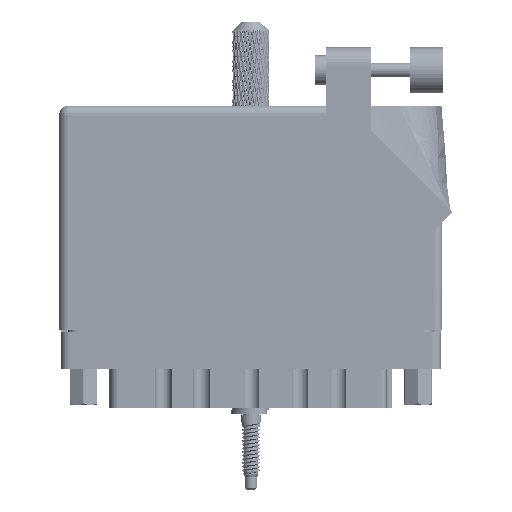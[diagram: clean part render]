
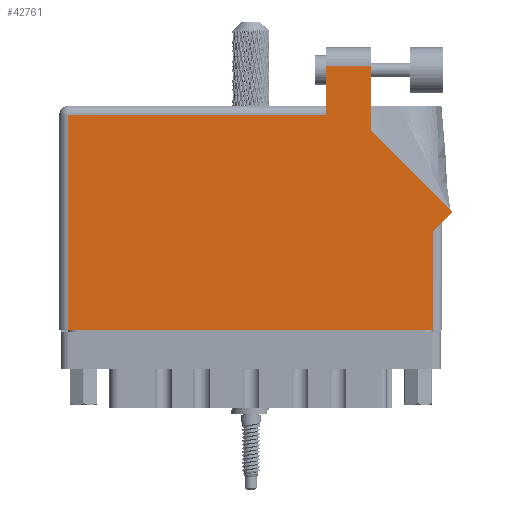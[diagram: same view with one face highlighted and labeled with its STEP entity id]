
A CAD part, front view. The second image highlights one B-rep face of the part: STEP entity #42761.
In plain terms, the highlighted face is planar.
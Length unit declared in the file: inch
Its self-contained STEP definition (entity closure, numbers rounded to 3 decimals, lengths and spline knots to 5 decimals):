
#889 = EDGE_CURVE ( 'NONE', #125285, #100103, #97054, .T. ) ;
#2261 = CARTESIAN_POINT ( 'NONE',  ( 0.062, 1.468, 0. ) ) ;
#2475 = DIRECTION ( 'NONE',  ( 0., -1., 0. ) ) ;
#2908 = CARTESIAN_POINT ( 'NONE',  ( 0.062, 0., 0. ) ) ;
#2923 = CARTESIAN_POINT ( 'NONE',  ( 2.55, 0.675, 0. ) ) ;
#3176 = CARTESIAN_POINT ( 'NONE',  ( 0., 1.53, 0. ) ) ;
#3602 = DIRECTION ( 'NONE',  ( -1., 0., 0. ) ) ;
#3746 = CARTESIAN_POINT ( 'NONE',  ( 1.819, 1.468, 0. ) ) ;
#4443 = CARTESIAN_POINT ( 'NONE',  ( 2.126, 1.36442, 0. ) ) ;
#5209 = DIRECTION ( 'NONE',  ( -0.707, 0.707, 0. ) ) ;
#12497 = LINE ( 'NONE', #119023, #41868 ) ;
#13631 = VECTOR ( 'NONE', #2475, 39.37008 ) ;
#15445 = LINE ( 'NONE', #98845, #117374 ) ;
#19598 = VECTOR ( 'NONE', #89529, 39.37008 ) ;
#20629 = DIRECTION ( 'NONE',  ( 0., 1., 0. ) ) ;
#27880 = LINE ( 'NONE', #84916, #81820 ) ;
#28435 = VERTEX_POINT ( 'NONE', #3746 ) ;
#29149 = EDGE_CURVE ( 'NONE', #54932, #73331, #53406, .T. ) ;
#33263 = VERTEX_POINT ( 'NONE', #53024 ) ;
#33855 = VERTEX_POINT ( 'NONE', #74916 ) ;
#35465 = CARTESIAN_POINT ( 'NONE',  ( 0., 1.468, 0. ) ) ;
#35721 = DIRECTION ( 'NONE',  ( 0.707, 0.707, 0. ) ) ;
#38159 = LINE ( 'NONE', #60083, #19598 ) ;
#38799 = ORIENTED_EDGE ( 'NONE', *, *, #50489, .T. ) ;
#39021 = LINE ( 'NONE', #52454, #88460 ) ;
#41401 = ORIENTED_EDGE ( 'NONE', *, *, #29149, .T. ) ;
#41868 = VECTOR ( 'NONE', #80626, 39.37008 ) ;
#42761 = ADVANCED_FACE ( 'NONE', ( #68547 ), #42949, .F. ) ;
#42949 = PLANE ( 'NONE',  #79005 ) ;
#49783 = VERTEX_POINT ( 'NONE', #2923 ) ;
#50489 = EDGE_CURVE ( 'NONE', #33263, #73759, #39021, .T. ) ;
#51599 = EDGE_CURVE ( 'NONE', #100103, #33855, #12497, .T. ) ;
#52454 = CARTESIAN_POINT ( 'NONE',  ( 1.819, 1.805, 0. ) ) ;
#53024 = CARTESIAN_POINT ( 'NONE',  ( 2.126, 1.805, 0. ) ) ;
#53406 = LINE ( 'NONE', #113147, #98224 ) ;
#54932 = VERTEX_POINT ( 'NONE', #63872 ) ;
#56821 = CARTESIAN_POINT ( 'NONE',  ( 1.819, 1.805, 0. ) ) ;
#57573 = ORIENTED_EDGE ( 'NONE', *, *, #118923, .T. ) ;
#60083 = CARTESIAN_POINT ( 'NONE',  ( 2.126, 1.36442, 0. ) ) ;
#63872 = CARTESIAN_POINT ( 'NONE',  ( 2.68271, 0.80771, 0. ) ) ;
#68547 = FACE_OUTER_BOUND ( 'NONE', #113799, .T. ) ;
#70097 = ORIENTED_EDGE ( 'NONE', *, *, #118599, .T. ) ;
#70231 = CARTESIAN_POINT ( 'NONE',  ( 2.55, 0.737, 0. ) ) ;
#73331 = VERTEX_POINT ( 'NONE', #4443 ) ;
#73759 = VERTEX_POINT ( 'NONE', #56821 ) ;
#74916 = CARTESIAN_POINT ( 'NONE',  ( 2.55, 0., 0. ) ) ;
#79005 = AXIS2_PLACEMENT_3D ( 'NONE', #3176, #120670, #3602 ) ;
#80626 = DIRECTION ( 'NONE',  ( 1., 0., 0. ) ) ;
#81820 = VECTOR ( 'NONE', #35721, 39.37008 ) ;
#82724 = VECTOR ( 'NONE', #20629, 39.37008 ) ;
#83279 = ORIENTED_EDGE ( 'NONE', *, *, #86297, .T. ) ;
#83974 = EDGE_CURVE ( 'NONE', #33855, #49783, #108997, .T. ) ;
#84240 = ORIENTED_EDGE ( 'NONE', *, *, #51599, .T. ) ;
#84916 = CARTESIAN_POINT ( 'NONE',  ( 2.612, 0.737, 0. ) ) ;
#86297 = EDGE_CURVE ( 'NONE', #28435, #125285, #99447, .T. ) ;
#88460 = VECTOR ( 'NONE', #121972, 39.37008 ) ;
#88885 = DIRECTION ( 'NONE',  ( 0., -1., 0. ) ) ;
#89529 = DIRECTION ( 'NONE',  ( 0., 1., 0. ) ) ;
#93829 = EDGE_CURVE ( 'NONE', #73331, #33263, #38159, .T. ) ;
#97054 = LINE ( 'NONE', #2908, #13631 ) ;
#98224 = VECTOR ( 'NONE', #5209, 39.37008 ) ;
#98845 = CARTESIAN_POINT ( 'NONE',  ( 1.819, 1.53, 0. ) ) ;
#99447 = LINE ( 'NONE', #35465, #102511 ) ;
#100103 = VERTEX_POINT ( 'NONE', #102044 ) ;
#102044 = CARTESIAN_POINT ( 'NONE',  ( 0.062, 0., 0. ) ) ;
#102511 = VECTOR ( 'NONE', #125669, 39.37008 ) ;
#108997 = LINE ( 'NONE', #70231, #82724 ) ;
#110341 = ORIENTED_EDGE ( 'NONE', *, *, #889, .T. ) ;
#113147 = CARTESIAN_POINT ( 'NONE',  ( 2.68271, 0.80771, 0. ) ) ;
#113407 = ORIENTED_EDGE ( 'NONE', *, *, #83974, .T. ) ;
#113799 = EDGE_LOOP ( 'NONE', ( #120522, #38799, #70097, #83279, #110341, #84240, #113407, #57573, #41401 ) ) ;
#117374 = VECTOR ( 'NONE', #88885, 39.37008 ) ;
#118599 = EDGE_CURVE ( 'NONE', #73759, #28435, #15445, .T. ) ;
#118923 = EDGE_CURVE ( 'NONE', #49783, #54932, #27880, .T. ) ;
#119023 = CARTESIAN_POINT ( 'NONE',  ( 0., 0., 0. ) ) ;
#120522 = ORIENTED_EDGE ( 'NONE', *, *, #93829, .T. ) ;
#120670 = DIRECTION ( 'NONE',  ( 0., 0., -1. ) ) ;
#121972 = DIRECTION ( 'NONE',  ( -1., 0., 0. ) ) ;
#125285 = VERTEX_POINT ( 'NONE', #2261 ) ;
#125669 = DIRECTION ( 'NONE',  ( -1., 0., 0. ) ) ;
